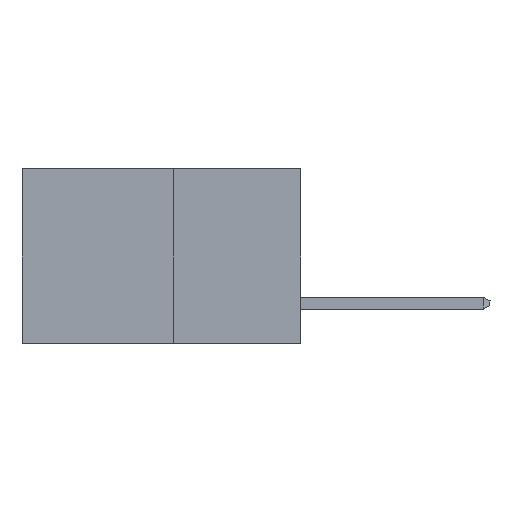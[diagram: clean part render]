
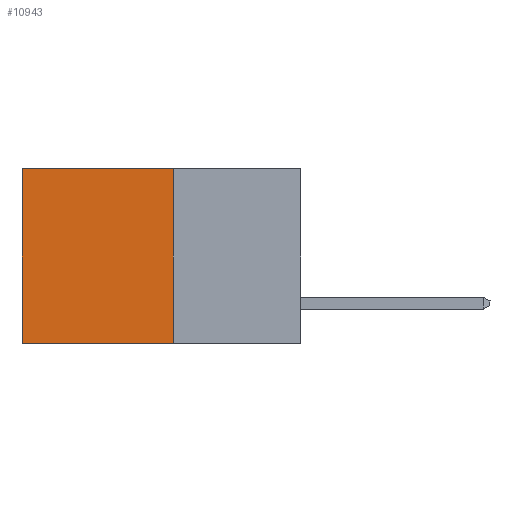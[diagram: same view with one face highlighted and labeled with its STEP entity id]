
A CAD part, left-side view. The second image highlights one B-rep face of the part: STEP entity #10943.
In plain terms, the highlighted planar face has unit normal (-1, 0, 0).
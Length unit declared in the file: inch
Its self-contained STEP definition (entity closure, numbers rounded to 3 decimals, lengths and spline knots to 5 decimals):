
#267 = ORIENTED_EDGE ( 'NONE', *, *, #6192, .T. ) ;
#684 = CARTESIAN_POINT ( 'NONE',  ( 0.277, 0.27, -0.37 ) ) ;
#733 = EDGE_CURVE ( 'NONE', #4119, #9273, #11589, .T. ) ;
#854 = ORIENTED_EDGE ( 'NONE', *, *, #8564, .T. ) ;
#1255 = DIRECTION ( 'NONE',  ( 1., 0., 0. ) ) ;
#1380 = EDGE_LOOP ( 'NONE', ( #854, #1790, #10660, #267 ) ) ;
#1414 = FACE_OUTER_BOUND ( 'NONE', #1380, .T. ) ;
#1653 = CARTESIAN_POINT ( 'NONE',  ( 0.277, 0.59, 0. ) ) ;
#1790 = ORIENTED_EDGE ( 'NONE', *, *, #733, .F. ) ;
#1918 = CARTESIAN_POINT ( 'NONE',  ( 0.277, 0.59, -0.37 ) ) ;
#2322 = LINE ( 'NONE', #1918, #7486 ) ;
#2523 = DIRECTION ( 'NONE',  ( 0., 1., 0. ) ) ;
#3274 = CARTESIAN_POINT ( 'NONE',  ( 0.277, 0.27, 0. ) ) ;
#3516 = LINE ( 'NONE', #12291, #8683 ) ;
#4119 = VERTEX_POINT ( 'NONE', #684 ) ;
#5298 = CARTESIAN_POINT ( 'NONE',  ( 0.277, 0.27, -0.37 ) ) ;
#6192 = EDGE_CURVE ( 'NONE', #6358, #13050, #12808, .T. ) ;
#6358 = VERTEX_POINT ( 'NONE', #3274 ) ;
#6828 = CARTESIAN_POINT ( 'NONE',  ( 0.277, 0.59, -0.37 ) ) ;
#6905 = EDGE_CURVE ( 'NONE', #6358, #4119, #3516, .T. ) ;
#7100 = VECTOR ( 'NONE', #12260, 39.37008 ) ;
#7224 = DIRECTION ( 'NONE',  ( 0., 0., -1. ) ) ;
#7419 = CARTESIAN_POINT ( 'NONE',  ( 0.277, 0.27, -0.37 ) ) ;
#7486 = VECTOR ( 'NONE', #11181, 39.37008 ) ;
#8196 = CARTESIAN_POINT ( 'NONE',  ( 0.277, 0.27, 0. ) ) ;
#8465 = DIRECTION ( 'NONE',  ( 0., 0., -1. ) ) ;
#8564 = EDGE_CURVE ( 'NONE', #13050, #9273, #2322, .T. ) ;
#8683 = VECTOR ( 'NONE', #7224, 39.37008 ) ;
#8908 = VECTOR ( 'NONE', #2523, 39.37008 ) ;
#9273 = VERTEX_POINT ( 'NONE', #6828 ) ;
#10660 = ORIENTED_EDGE ( 'NONE', *, *, #6905, .F. ) ;
#10943 = ADVANCED_FACE ( 'NONE', ( #1414 ), #12431, .F. ) ;
#11181 = DIRECTION ( 'NONE',  ( 0., 0., -1. ) ) ;
#11589 = LINE ( 'NONE', #5298, #8908 ) ;
#12078 = AXIS2_PLACEMENT_3D ( 'NONE', #7419, #1255, #8465 ) ;
#12260 = DIRECTION ( 'NONE',  ( 0., 1., 0. ) ) ;
#12291 = CARTESIAN_POINT ( 'NONE',  ( 0.277, 0.27, -0.37 ) ) ;
#12431 = PLANE ( 'NONE',  #12078 ) ;
#12808 = LINE ( 'NONE', #8196, #7100 ) ;
#13050 = VERTEX_POINT ( 'NONE', #1653 ) ;
